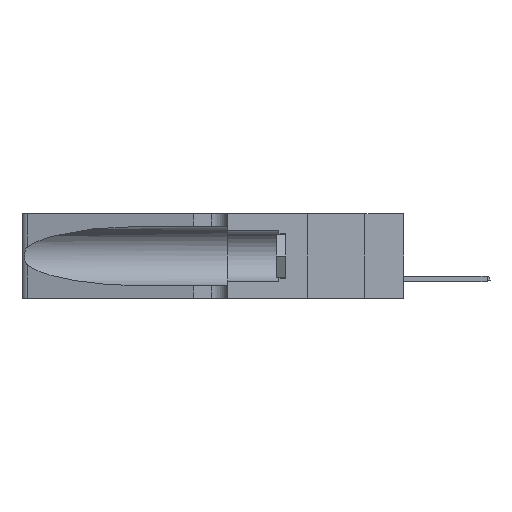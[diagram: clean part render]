
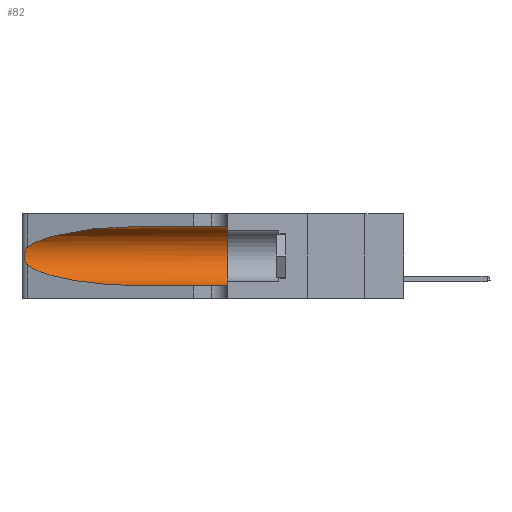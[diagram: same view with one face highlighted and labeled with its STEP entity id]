
A CAD part, left-side view. The second image highlights one B-rep face of the part: STEP entity #82.
In plain terms, the highlighted cylindrical face has radius 3.308 mm (diameter 6.617 mm), a partial arc.
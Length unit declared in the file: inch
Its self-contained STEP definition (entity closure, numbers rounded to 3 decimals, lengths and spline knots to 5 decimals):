
#1 = CARTESIAN_POINT ( 'NONE',  ( 0.1305, 1.61858, 0.185 ) ) ;
#82 = ADVANCED_FACE ( 'NONE', ( #28815 ), #19184, .F. ) ;
#462 = CARTESIAN_POINT ( 'NONE',  ( 0.1305, 0.72297, 0.31525 ) ) ;
#540 = EDGE_LOOP ( 'NONE', ( #32521, #32335, #8243, #19656, #29367, #10884 ) ) ;
#1201 = CARTESIAN_POINT ( 'NONE',  ( 0.25856, 1.23593, 0.16098 ) ) ;
#2736 = LINE ( 'NONE', #18851, #20257 ) ;
#3162 = EDGE_CURVE ( 'NONE', #17839, #31489, #12508, .T. ) ;
#3194 = CARTESIAN_POINT ( 'NONE',  ( 0.1305, 0.72297, 0.05475 ) ) ;
#4018 = CARTESIAN_POINT ( 'NONE',  ( 0.25555, 1.22993, 0.14849 ) ) ;
#4386 = CARTESIAN_POINT ( 'NONE',  ( 0.26017, 1.23833, 0.17102 ) ) ;
#5031 = CARTESIAN_POINT ( 'NONE',  ( 0.25487, 1.22718, 0.22369 ) ) ;
#5212 = EDGE_CURVE ( 'NONE', #17694, #6942, #8024, .T. ) ;
#5498 = EDGE_CURVE ( 'NONE', #17839, #31776, #2736, .T. ) ;
#6246 = CARTESIAN_POINT ( 'NONE',  ( 0.2373, 1.15595, 0.08982 ) ) ;
#6637 = DIRECTION ( 'NONE',  ( 0., 1., 0. ) ) ;
#6942 = VERTEX_POINT ( 'NONE', #13655 ) ;
#8024 = LINE ( 'NONE', #13626, #8843 ) ;
#8243 = ORIENTED_EDGE ( 'NONE', *, *, #30595, .T. ) ;
#8498 = CARTESIAN_POINT ( 'NONE',  ( 0.1305, 0.72297, 0.05475 ) ) ;
#8617 = EDGE_CURVE ( 'NONE', #31489, #27286, #26733, .T. ) ;
#8843 = VECTOR ( 'NONE', #14797, 39.37008 ) ;
#9080 = CARTESIAN_POINT ( 'NONE',  ( 0.25487, 1.22718, 0.14631 ) ) ;
#9935 = CARTESIAN_POINT ( 'NONE',  ( 0.25555, 1.22994, 0.2215 ) ) ;
#9964 = CARTESIAN_POINT ( 'NONE',  ( 0.18966, 0.96281, 0.31525 ) ) ;
#10884 = ORIENTED_EDGE ( 'NONE', *, *, #5498, .F. ) ;
#11913 = CARTESIAN_POINT ( 'NONE',  ( 0.1305, 0.35, 0.185 ) ) ;
#12508 =( BOUNDED_CURVE ( )  B_SPLINE_CURVE ( 3, ( #18547, #9964, #24935, #5031 ),
 .UNSPECIFIED., .F., .T. ) 
 B_SPLINE_CURVE_WITH_KNOTS ( ( 4, 4 ),
 ( 1.5708, 2.84003 ),
 .UNSPECIFIED. ) 
 CURVE ( )  GEOMETRIC_REPRESENTATION_ITEM ( )  RATIONAL_B_SPLINE_CURVE ( ( 1., 0.87, 0.87, 1. ) ) 
 REPRESENTATION_ITEM ( '' )  );
#13626 = CARTESIAN_POINT ( 'NONE',  ( 0.1305, 1.61858, 0.05475 ) ) ;
#13655 = CARTESIAN_POINT ( 'NONE',  ( 0.1305, 0.35, 0.05475 ) ) ;
#14543 = DIRECTION ( 'NONE',  ( 0., 0., -1. ) ) ;
#14797 = DIRECTION ( 'NONE',  ( 0., -1., 0. ) ) ;
#15684 = CARTESIAN_POINT ( 'NONE',  ( 0.25787, 1.23484, 0.2124 ) ) ;
#17694 = VERTEX_POINT ( 'NONE', #8498 ) ;
#17780 = EDGE_CURVE ( 'NONE', #31776, #6942, #25712, .T. ) ;
#17839 = VERTEX_POINT ( 'NONE', #462 ) ;
#18147 = CARTESIAN_POINT ( 'NONE',  ( 0.25487, 1.22718, 0.14631 ) ) ;
#18255 = CARTESIAN_POINT ( 'NONE',  ( 0.25854, 1.2359, 0.20912 ) ) ;
#18547 = CARTESIAN_POINT ( 'NONE',  ( 0.1305, 0.72297, 0.31525 ) ) ;
#18851 = CARTESIAN_POINT ( 'NONE',  ( 0.1305, 1.61858, 0.31525 ) ) ;
#19184 = CYLINDRICAL_SURFACE ( 'NONE', #35720, 0.13025 ) ;
#19656 = ORIENTED_EDGE ( 'NONE', *, *, #5212, .T. ) ;
#20257 = VECTOR ( 'NONE', #21686, 39.37008 ) ;
#21237 = CARTESIAN_POINT ( 'NONE',  ( 0.26075, 1.23896, 0.178 ) ) ;
#21686 = DIRECTION ( 'NONE',  ( 0., -1., 0. ) ) ;
#22570 = DIRECTION ( 'NONE',  ( 0., -1., 0. ) ) ;
#23203 = DIRECTION ( 'NONE',  ( 0., 0., 1. ) ) ;
#24055 = CARTESIAN_POINT ( 'NONE',  ( 0.25487, 1.22718, 0.14631 ) ) ;
#24935 = CARTESIAN_POINT ( 'NONE',  ( 0.2373, 1.15595, 0.28018 ) ) ;
#25518 = CARTESIAN_POINT ( 'NONE',  ( 0.1305, 0.35, 0.31525 ) ) ;
#25712 = CIRCLE ( 'NONE', #31636, 0.13025 ) ;
#26521 = CARTESIAN_POINT ( 'NONE',  ( 0.25639, 1.23184, 0.21858 ) ) ;
#26699 = CARTESIAN_POINT ( 'NONE',  ( 0.25487, 1.22718, 0.22369 ) ) ;
#26733 = B_SPLINE_CURVE_WITH_KNOTS ( 'NONE', 3,
 ( #35221, #9935, #26521, #15684, #18255, #29581, #32416, #21237, #4386, #1201, #29697, #29320, #4018, #24055 ),
 .UNSPECIFIED., .F., .F.,
 ( 4, 2, 2, 2, 2, 2, 4 ),
 ( 0., 0.00027, 0.00053, 0.00107, 0.0016, 0.00187, 0.00214 ),
 .UNSPECIFIED. ) ;
#27286 = VERTEX_POINT ( 'NONE', #18147 ) ;
#28815 = FACE_OUTER_BOUND ( 'NONE', #540, .T. ) ;
#29320 = CARTESIAN_POINT ( 'NONE',  ( 0.25639, 1.23186, 0.15144 ) ) ;
#29367 = ORIENTED_EDGE ( 'NONE', *, *, #17780, .F. ) ;
#29581 = CARTESIAN_POINT ( 'NONE',  ( 0.26018, 1.23835, 0.19895 ) ) ;
#29697 = CARTESIAN_POINT ( 'NONE',  ( 0.25789, 1.23486, 0.15765 ) ) ;
#30595 = EDGE_CURVE ( 'NONE', #27286, #17694, #35477, .T. ) ;
#31197 = CARTESIAN_POINT ( 'NONE',  ( 0.18966, 0.96281, 0.05475 ) ) ;
#31489 = VERTEX_POINT ( 'NONE', #26699 ) ;
#31636 = AXIS2_PLACEMENT_3D ( 'NONE', #11913, #6637, #23203 ) ;
#31776 = VERTEX_POINT ( 'NONE', #25518 ) ;
#32335 = ORIENTED_EDGE ( 'NONE', *, *, #8617, .T. ) ;
#32416 = CARTESIAN_POINT ( 'NONE',  ( 0.26075, 1.23896, 0.19203 ) ) ;
#32521 = ORIENTED_EDGE ( 'NONE', *, *, #3162, .T. ) ;
#35221 = CARTESIAN_POINT ( 'NONE',  ( 0.25487, 1.22718, 0.22369 ) ) ;
#35477 =( BOUNDED_CURVE ( )  B_SPLINE_CURVE ( 3, ( #9080, #6246, #31197, #3194 ),
 .UNSPECIFIED., .F., .T. ) 
 B_SPLINE_CURVE_WITH_KNOTS ( ( 4, 4 ),
 ( 3.44316, 4.71239 ),
 .UNSPECIFIED. ) 
 CURVE ( )  GEOMETRIC_REPRESENTATION_ITEM ( )  RATIONAL_B_SPLINE_CURVE ( ( 1., 0.87, 0.87, 1. ) ) 
 REPRESENTATION_ITEM ( '' )  );
#35720 = AXIS2_PLACEMENT_3D ( 'NONE', #1, #22570, #14543 ) ;
